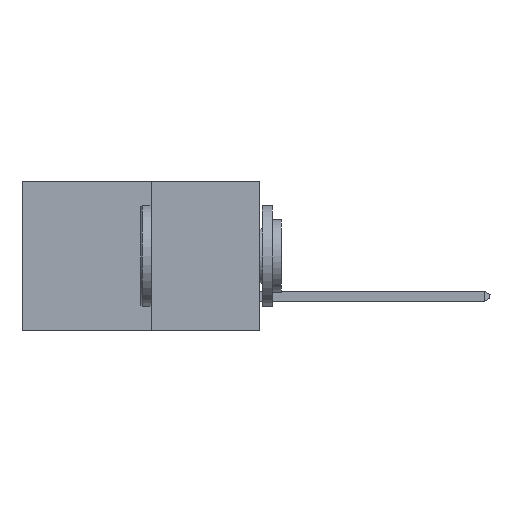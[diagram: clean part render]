
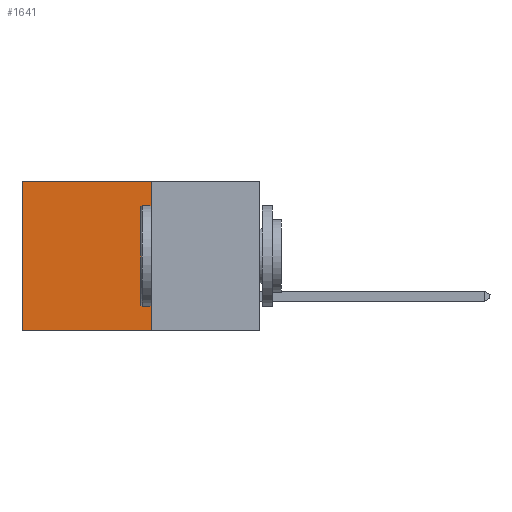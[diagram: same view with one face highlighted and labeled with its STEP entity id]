
A CAD part, left-side view. The second image highlights one B-rep face of the part: STEP entity #1641.
In plain terms, the highlighted planar face has unit normal (-1, 0, 0).
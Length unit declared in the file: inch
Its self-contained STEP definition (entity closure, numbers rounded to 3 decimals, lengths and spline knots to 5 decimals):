
#1641 = ADVANCED_FACE ( 'NONE', ( #24225 ), #17173, .F. ) ;
#2434 = LINE ( 'NONE', #26791, #4067 ) ;
#2467 = DIRECTION ( 'NONE',  ( 0., 1., 0. ) ) ;
#3361 = CARTESIAN_POINT ( 'NONE',  ( 0.277, 0.27, -0.37 ) ) ;
#3700 = LINE ( 'NONE', #3361, #9112 ) ;
#4067 = VECTOR ( 'NONE', #5769, 39.37008 ) ;
#4105 = LINE ( 'NONE', #27454, #30350 ) ;
#4701 = CARTESIAN_POINT ( 'NONE',  ( 0.277, 0.59, 0. ) ) ;
#5252 = EDGE_CURVE ( 'NONE', #12015, #11887, #3700, .T. ) ;
#5769 = DIRECTION ( 'NONE',  ( 0., 1., 0. ) ) ;
#9112 = VECTOR ( 'NONE', #2467, 39.37008 ) ;
#11364 = EDGE_CURVE ( 'NONE', #22458, #18079, #2434, .T. ) ;
#11550 = EDGE_CURVE ( 'NONE', #18079, #11887, #4105, .T. ) ;
#11887 = VERTEX_POINT ( 'NONE', #16200 ) ;
#12015 = VERTEX_POINT ( 'NONE', #16767 ) ;
#14489 = DIRECTION ( 'NONE',  ( 0., 0., -1. ) ) ;
#15292 = CARTESIAN_POINT ( 'NONE',  ( 0.277, 0.27, -0.37 ) ) ;
#16200 = CARTESIAN_POINT ( 'NONE',  ( 0.277, 0.59, -0.37 ) ) ;
#16304 = DIRECTION ( 'NONE',  ( 0., 0., -1. ) ) ;
#16445 = DIRECTION ( 'NONE',  ( 1., 0., 0. ) ) ;
#16707 = CARTESIAN_POINT ( 'NONE',  ( 0.277, 0.27, -0.37 ) ) ;
#16767 = CARTESIAN_POINT ( 'NONE',  ( 0.277, 0.27, -0.37 ) ) ;
#17141 = ORIENTED_EDGE ( 'NONE', *, *, #11364, .T. ) ;
#17173 = PLANE ( 'NONE',  #24691 ) ;
#17913 = DIRECTION ( 'NONE',  ( 0., 0., -1. ) ) ;
#18079 = VERTEX_POINT ( 'NONE', #4701 ) ;
#18948 = VECTOR ( 'NONE', #17913, 39.37008 ) ;
#20616 = LINE ( 'NONE', #15292, #18948 ) ;
#22458 = VERTEX_POINT ( 'NONE', #28894 ) ;
#24225 = FACE_OUTER_BOUND ( 'NONE', #27533, .T. ) ;
#24691 = AXIS2_PLACEMENT_3D ( 'NONE', #16707, #16445, #16304 ) ;
#26791 = CARTESIAN_POINT ( 'NONE',  ( 0.277, 0.27, 0. ) ) ;
#27454 = CARTESIAN_POINT ( 'NONE',  ( 0.277, 0.59, -0.37 ) ) ;
#27533 = EDGE_LOOP ( 'NONE', ( #27967, #29756, #32512, #17141 ) ) ;
#27967 = ORIENTED_EDGE ( 'NONE', *, *, #11550, .T. ) ;
#28894 = CARTESIAN_POINT ( 'NONE',  ( 0.277, 0.27, 0. ) ) ;
#29756 = ORIENTED_EDGE ( 'NONE', *, *, #5252, .F. ) ;
#29797 = EDGE_CURVE ( 'NONE', #22458, #12015, #20616, .T. ) ;
#30350 = VECTOR ( 'NONE', #14489, 39.37008 ) ;
#32512 = ORIENTED_EDGE ( 'NONE', *, *, #29797, .F. ) ;
